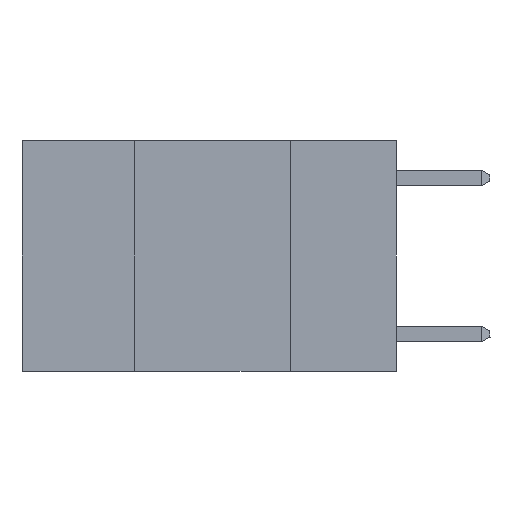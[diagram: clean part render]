
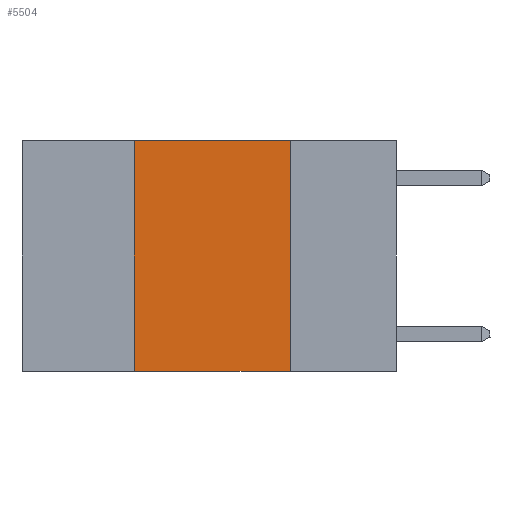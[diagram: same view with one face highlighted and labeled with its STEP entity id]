
A CAD part, left-side view. The second image highlights one B-rep face of the part: STEP entity #5504.
In plain terms, the highlighted planar face has unit normal (-1, 0, 0).
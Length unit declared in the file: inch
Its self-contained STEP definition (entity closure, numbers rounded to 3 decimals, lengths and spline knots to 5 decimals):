
#24 = VERTEX_POINT ( 'NONE', #6157 ) ;
#735 = DIRECTION ( 'NONE',  ( 1., 0., 0. ) ) ;
#1537 = DIRECTION ( 'NONE',  ( 0., -1., 0. ) ) ;
#2548 = ORIENTED_EDGE ( 'NONE', *, *, #9317, .T. ) ;
#2914 = DIRECTION ( 'NONE',  ( 0., -1., 0. ) ) ;
#3445 = CARTESIAN_POINT ( 'NONE',  ( 0., 0.17, 0. ) ) ;
#3923 = EDGE_LOOP ( 'NONE', ( #7599, #6940, #15883, #2548 ) ) ;
#5504 = ADVANCED_FACE ( 'NONE', ( #10382 ), #11864, .F. ) ;
#6157 = CARTESIAN_POINT ( 'NONE',  ( 0., 0.17, -0.37 ) ) ;
#6940 = ORIENTED_EDGE ( 'NONE', *, *, #11603, .F. ) ;
#7414 = CARTESIAN_POINT ( 'NONE',  ( 0., 0.42, -0.37 ) ) ;
#7599 = ORIENTED_EDGE ( 'NONE', *, *, #14464, .F. ) ;
#7692 = DIRECTION ( 'NONE',  ( 0., 0., -1. ) ) ;
#8680 = LINE ( 'NONE', #3445, #17327 ) ;
#9317 = EDGE_CURVE ( 'NONE', #13155, #24, #14048, .T. ) ;
#9473 = CARTESIAN_POINT ( 'NONE',  ( 0., 0.42, 0. ) ) ;
#9522 = AXIS2_PLACEMENT_3D ( 'NONE', #16283, #735, #7692 ) ;
#9727 = DIRECTION ( 'NONE',  ( 0., 0., 1. ) ) ;
#10382 = FACE_OUTER_BOUND ( 'NONE', #3923, .T. ) ;
#11603 = EDGE_CURVE ( 'NONE', #12685, #11805, #12407, .T. ) ;
#11805 = VERTEX_POINT ( 'NONE', #13214 ) ;
#11864 = PLANE ( 'NONE',  #9522 ) ;
#12407 = LINE ( 'NONE', #18111, #13068 ) ;
#12685 = VERTEX_POINT ( 'NONE', #17238 ) ;
#13017 = DIRECTION ( 'NONE',  ( 0., 0., -1. ) ) ;
#13068 = VECTOR ( 'NONE', #1537, 39.37008 ) ;
#13155 = VERTEX_POINT ( 'NONE', #7414 ) ;
#13214 = CARTESIAN_POINT ( 'NONE',  ( 0., 0.17, 0. ) ) ;
#13718 = LINE ( 'NONE', #9473, #14669 ) ;
#14048 = LINE ( 'NONE', #18018, #17756 ) ;
#14464 = EDGE_CURVE ( 'NONE', #11805, #24, #8680, .T. ) ;
#14669 = VECTOR ( 'NONE', #9727, 39.37008 ) ;
#15083 = EDGE_CURVE ( 'NONE', #13155, #12685, #13718, .T. ) ;
#15883 = ORIENTED_EDGE ( 'NONE', *, *, #15083, .F. ) ;
#16283 = CARTESIAN_POINT ( 'NONE',  ( 0., 0.6, 0. ) ) ;
#17238 = CARTESIAN_POINT ( 'NONE',  ( 0., 0.42, 0. ) ) ;
#17327 = VECTOR ( 'NONE', #13017, 39.37008 ) ;
#17756 = VECTOR ( 'NONE', #2914, 39.37008 ) ;
#18018 = CARTESIAN_POINT ( 'NONE',  ( 0., 0.6, -0.37 ) ) ;
#18111 = CARTESIAN_POINT ( 'NONE',  ( 0., 0.6, 0. ) ) ;
